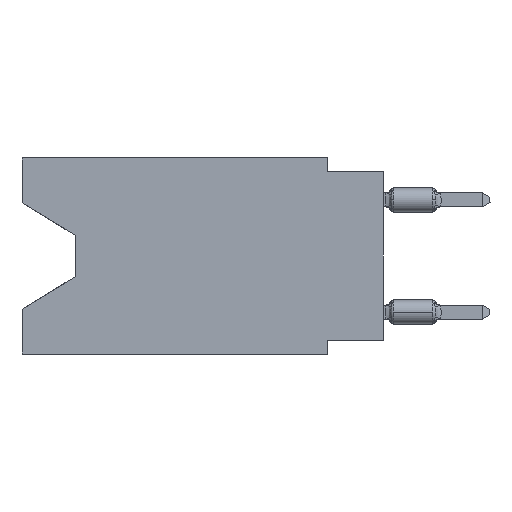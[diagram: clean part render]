
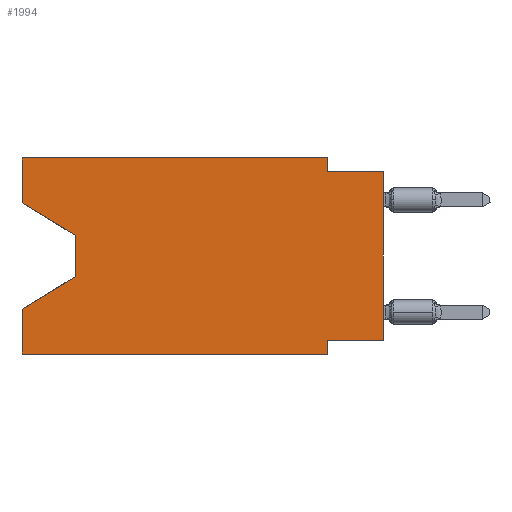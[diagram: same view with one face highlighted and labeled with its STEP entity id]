
A CAD part, left-side view. The second image highlights one B-rep face of the part: STEP entity #1994.
In plain terms, the highlighted planar face has unit normal (-1, 0, 0).
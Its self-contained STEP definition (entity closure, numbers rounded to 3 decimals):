
#213 = DIRECTION ( 'NONE',  ( 0., 0.855, -0.519 ) ) ;
#456 = DIRECTION ( 'NONE',  ( 0., -0.855, -0.519 ) ) ;
#620 = ORIENTED_EDGE ( 'NONE', *, *, #49860, .T. ) ;
#1056 = VECTOR ( 'NONE', #456, 1000. ) ;
#1065 = VERTEX_POINT ( 'NONE', #6560 ) ;
#1119 = CARTESIAN_POINT ( 'NONE',  ( 0., 0., 0. ) ) ;
#1551 = LINE ( 'NONE', #13231, #18743 ) ;
#1994 = ADVANCED_FACE ( 'NONE', ( #42001 ), #37723, .F. ) ;
#2008 = EDGE_CURVE ( 'NONE', #46303, #27271, #50816, .T. ) ;
#2142 = DIRECTION ( 'NONE',  ( 0., 0., -1. ) ) ;
#2545 = DIRECTION ( 'NONE',  ( 0., 0., -1. ) ) ;
#3546 = VECTOR ( 'NONE', #213, 1000. ) ;
#3882 = LINE ( 'NONE', #21262, #1056 ) ;
#4462 = VERTEX_POINT ( 'NONE', #38938 ) ;
#6560 = CARTESIAN_POINT ( 'NONE',  ( 0., 16.383, 0. ) ) ;
#6783 = EDGE_CURVE ( 'NONE', #31196, #52791, #7646, .T. ) ;
#7549 = DIRECTION ( 'NONE',  ( 0., 1., 0. ) ) ;
#7646 = LINE ( 'NONE', #33015, #35298 ) ;
#10045 = VECTOR ( 'NONE', #7549, 1000. ) ;
#10101 = CARTESIAN_POINT ( 'NONE',  ( 0., 16.383, -8.89 ) ) ;
#10659 = DIRECTION ( 'NONE',  ( 0., 0., 1. ) ) ;
#11076 = EDGE_CURVE ( 'NONE', #4462, #46303, #41202, .T. ) ;
#11224 = CARTESIAN_POINT ( 'NONE',  ( 0., 2.54, -0.635 ) ) ;
#11321 = ORIENTED_EDGE ( 'NONE', *, *, #26450, .T. ) ;
#11786 = CARTESIAN_POINT ( 'NONE',  ( 0., 2.54, -8.89 ) ) ;
#12986 = ORIENTED_EDGE ( 'NONE', *, *, #42210, .F. ) ;
#13231 = CARTESIAN_POINT ( 'NONE',  ( 0., 16.383, 0. ) ) ;
#13516 = CARTESIAN_POINT ( 'NONE',  ( 0., 16.383, 0. ) ) ;
#15733 = DIRECTION ( 'NONE',  ( 0., -1., 0. ) ) ;
#16067 = CARTESIAN_POINT ( 'NONE',  ( 0., 13.97, -3.505 ) ) ;
#18181 = DIRECTION ( 'NONE',  ( 0., 0., 1. ) ) ;
#18346 = EDGE_CURVE ( 'NONE', #38639, #55750, #33651, .T. ) ;
#18743 = VECTOR ( 'NONE', #10659, 1000. ) ;
#18831 = ORIENTED_EDGE ( 'NONE', *, *, #19355, .F. ) ;
#18881 = ORIENTED_EDGE ( 'NONE', *, *, #11076, .F. ) ;
#19050 = ORIENTED_EDGE ( 'NONE', *, *, #39395, .T. ) ;
#19286 = CARTESIAN_POINT ( 'NONE',  ( 0., 16.383, -8.89 ) ) ;
#19355 = EDGE_CURVE ( 'NONE', #1065, #49984, #33795, .T. ) ;
#19636 = VECTOR ( 'NONE', #32396, 1000. ) ;
#20584 = EDGE_CURVE ( 'NONE', #4462, #55750, #52659, .T. ) ;
#20989 = ORIENTED_EDGE ( 'NONE', *, *, #28058, .F. ) ;
#21262 = CARTESIAN_POINT ( 'NONE',  ( 0., 16.383, -2.038 ) ) ;
#22107 = VECTOR ( 'NONE', #31825, 1000. ) ;
#22569 = VECTOR ( 'NONE', #30607, 1000. ) ;
#23625 = CARTESIAN_POINT ( 'NONE',  ( 0., 13.97, -5.385 ) ) ;
#24010 = CARTESIAN_POINT ( 'NONE',  ( 0., 0., -0.635 ) ) ;
#24318 = CARTESIAN_POINT ( 'NONE',  ( 0., 16.383, -2.038 ) ) ;
#26450 = EDGE_CURVE ( 'NONE', #53827, #31196, #3882, .T. ) ;
#26507 = CARTESIAN_POINT ( 'NONE',  ( 0., 0., -0.635 ) ) ;
#26692 = LINE ( 'NONE', #27247, #3546 ) ;
#27247 = CARTESIAN_POINT ( 'NONE',  ( 0., 13.97, -5.385 ) ) ;
#27271 = VERTEX_POINT ( 'NONE', #52441 ) ;
#28058 = EDGE_CURVE ( 'NONE', #49984, #38639, #39825, .T. ) ;
#30607 = DIRECTION ( 'NONE',  ( 0., 0., 1. ) ) ;
#31196 = VERTEX_POINT ( 'NONE', #16067 ) ;
#31825 = DIRECTION ( 'NONE',  ( 0., 0., -1. ) ) ;
#32396 = DIRECTION ( 'NONE',  ( 0., -1., 0. ) ) ;
#33015 = CARTESIAN_POINT ( 'NONE',  ( 0., 13.97, -3.505 ) ) ;
#33651 = LINE ( 'NONE', #24010, #36718 ) ;
#33795 = LINE ( 'NONE', #38357, #48245 ) ;
#35298 = VECTOR ( 'NONE', #2545, 1000. ) ;
#35382 = EDGE_LOOP ( 'NONE', ( #11321, #55462, #620, #12986, #19050, #46885, #18881, #39167, #37751, #20989, #18831, #39544 ) ) ;
#36042 = VERTEX_POINT ( 'NONE', #10101 ) ;
#36342 = CARTESIAN_POINT ( 'NONE',  ( 0., 2.54, -8.255 ) ) ;
#36718 = VECTOR ( 'NONE', #15733, 1000. ) ;
#37160 = DIRECTION ( 'NONE',  ( 1., 0., 0. ) ) ;
#37723 = PLANE ( 'NONE',  #37784 ) ;
#37751 = ORIENTED_EDGE ( 'NONE', *, *, #18346, .F. ) ;
#37784 = AXIS2_PLACEMENT_3D ( 'NONE', #41159, #37160, #2142 ) ;
#38357 = CARTESIAN_POINT ( 'NONE',  ( 0., 16.383, 0. ) ) ;
#38639 = VERTEX_POINT ( 'NONE', #11224 ) ;
#38938 = CARTESIAN_POINT ( 'NONE',  ( 0., 0., -8.255 ) ) ;
#39167 = ORIENTED_EDGE ( 'NONE', *, *, #20584, .T. ) ;
#39395 = EDGE_CURVE ( 'NONE', #36042, #27271, #41779, .T. ) ;
#39544 = ORIENTED_EDGE ( 'NONE', *, *, #40201, .F. ) ;
#39728 = LINE ( 'NONE', #13516, #22569 ) ;
#39825 = LINE ( 'NONE', #53204, #22107 ) ;
#40201 = EDGE_CURVE ( 'NONE', #53827, #1065, #1551, .T. ) ;
#41159 = CARTESIAN_POINT ( 'NONE',  ( 0., 16.383, 0. ) ) ;
#41202 = LINE ( 'NONE', #54293, #10045 ) ;
#41779 = LINE ( 'NONE', #19286, #19636 ) ;
#42001 = FACE_OUTER_BOUND ( 'NONE', #35382, .T. ) ;
#42210 = EDGE_CURVE ( 'NONE', #36042, #50769, #39728, .T. ) ;
#44515 = CARTESIAN_POINT ( 'NONE',  ( 0., 16.383, -6.852 ) ) ;
#46303 = VERTEX_POINT ( 'NONE', #36342 ) ;
#46563 = DIRECTION ( 'NONE',  ( 0., 0., -1. ) ) ;
#46885 = ORIENTED_EDGE ( 'NONE', *, *, #2008, .F. ) ;
#47475 = VECTOR ( 'NONE', #18181, 1000. ) ;
#47811 = VECTOR ( 'NONE', #46563, 1000. ) ;
#48245 = VECTOR ( 'NONE', #51179, 1000. ) ;
#49860 = EDGE_CURVE ( 'NONE', #52791, #50769, #26692, .T. ) ;
#49984 = VERTEX_POINT ( 'NONE', #50588 ) ;
#50588 = CARTESIAN_POINT ( 'NONE',  ( 0., 2.54, 0. ) ) ;
#50769 = VERTEX_POINT ( 'NONE', #44515 ) ;
#50816 = LINE ( 'NONE', #11786, #47811 ) ;
#51179 = DIRECTION ( 'NONE',  ( 0., -1., 0. ) ) ;
#52441 = CARTESIAN_POINT ( 'NONE',  ( 0., 2.54, -8.89 ) ) ;
#52659 = LINE ( 'NONE', #1119, #47475 ) ;
#52791 = VERTEX_POINT ( 'NONE', #23625 ) ;
#53204 = CARTESIAN_POINT ( 'NONE',  ( 0., 2.54, 0. ) ) ;
#53827 = VERTEX_POINT ( 'NONE', #24318 ) ;
#54293 = CARTESIAN_POINT ( 'NONE',  ( 0., 0., -8.255 ) ) ;
#55462 = ORIENTED_EDGE ( 'NONE', *, *, #6783, .T. ) ;
#55750 = VERTEX_POINT ( 'NONE', #26507 ) ;
